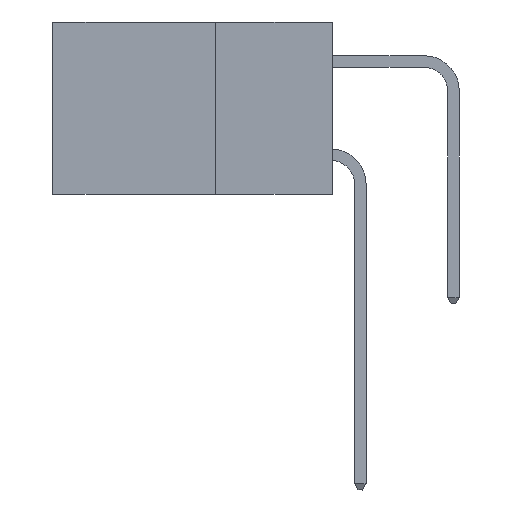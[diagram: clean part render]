
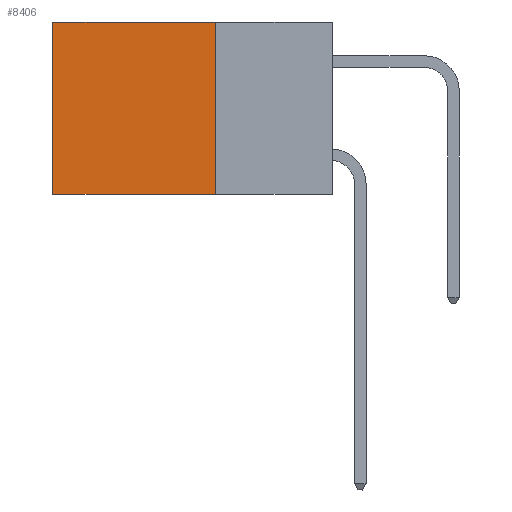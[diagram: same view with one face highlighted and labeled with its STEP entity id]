
A CAD part, left-side view. The second image highlights one B-rep face of the part: STEP entity #8406.
In plain terms, the highlighted planar face has unit normal (-1, 0, 0).
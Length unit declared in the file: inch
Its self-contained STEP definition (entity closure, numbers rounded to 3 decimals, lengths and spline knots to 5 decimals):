
#489 = DIRECTION ( 'NONE',  ( 0., 0., -1. ) ) ;
#794 = VERTEX_POINT ( 'NONE', #6489 ) ;
#1992 = EDGE_CURVE ( 'NONE', #14299, #3176, #11150, .T. ) ;
#3059 = VECTOR ( 'NONE', #6526, 39.37008 ) ;
#3176 = VERTEX_POINT ( 'NONE', #12737 ) ;
#4518 = CARTESIAN_POINT ( 'NONE',  ( 0.2615, 0.25, -0.37 ) ) ;
#4718 = EDGE_CURVE ( 'NONE', #21495, #794, #13265, .T. ) ;
#6334 = CARTESIAN_POINT ( 'NONE',  ( 0.2615, 0.6, -0.37 ) ) ;
#6380 = EDGE_LOOP ( 'NONE', ( #12446, #15449, #20182, #7622 ) ) ;
#6489 = CARTESIAN_POINT ( 'NONE',  ( 0.2615, 0.6, -0.37 ) ) ;
#6526 = DIRECTION ( 'NONE',  ( 0., 0., -1. ) ) ;
#7274 = PLANE ( 'NONE',  #21575 ) ;
#7622 = ORIENTED_EDGE ( 'NONE', *, *, #1992, .T. ) ;
#7727 = DIRECTION ( 'NONE',  ( 0., 1., 0. ) ) ;
#8406 = ADVANCED_FACE ( 'NONE', ( #12726 ), #7274, .F. ) ;
#8997 = DIRECTION ( 'NONE',  ( 1., 0., 0. ) ) ;
#10284 = DIRECTION ( 'NONE',  ( 0., 0., -1. ) ) ;
#10830 = CARTESIAN_POINT ( 'NONE',  ( 0.2615, 0.25, 0. ) ) ;
#11150 = LINE ( 'NONE', #17906, #19831 ) ;
#11304 = VECTOR ( 'NONE', #10284, 39.37008 ) ;
#12446 = ORIENTED_EDGE ( 'NONE', *, *, #16599, .T. ) ;
#12726 = FACE_OUTER_BOUND ( 'NONE', #6380, .T. ) ;
#12737 = CARTESIAN_POINT ( 'NONE',  ( 0.2615, 0.6, 0. ) ) ;
#13265 = LINE ( 'NONE', #4518, #16425 ) ;
#14299 = VERTEX_POINT ( 'NONE', #10830 ) ;
#15449 = ORIENTED_EDGE ( 'NONE', *, *, #4718, .F. ) ;
#16425 = VECTOR ( 'NONE', #20136, 39.37008 ) ;
#16599 = EDGE_CURVE ( 'NONE', #3176, #794, #22230, .T. ) ;
#17689 = CARTESIAN_POINT ( 'NONE',  ( 0.2615, 0.25, -0.37 ) ) ;
#17906 = CARTESIAN_POINT ( 'NONE',  ( 0.2615, 0.25, 0. ) ) ;
#19831 = VECTOR ( 'NONE', #7727, 39.37008 ) ;
#20136 = DIRECTION ( 'NONE',  ( 0., 1., 0. ) ) ;
#20182 = ORIENTED_EDGE ( 'NONE', *, *, #21010, .F. ) ;
#20823 = CARTESIAN_POINT ( 'NONE',  ( 0.2615, 0.25, -0.37 ) ) ;
#21010 = EDGE_CURVE ( 'NONE', #14299, #21495, #21670, .T. ) ;
#21214 = CARTESIAN_POINT ( 'NONE',  ( 0.2615, 0.25, -0.37 ) ) ;
#21495 = VERTEX_POINT ( 'NONE', #20823 ) ;
#21575 = AXIS2_PLACEMENT_3D ( 'NONE', #17689, #8997, #489 ) ;
#21670 = LINE ( 'NONE', #21214, #3059 ) ;
#22230 = LINE ( 'NONE', #6334, #11304 ) ;
